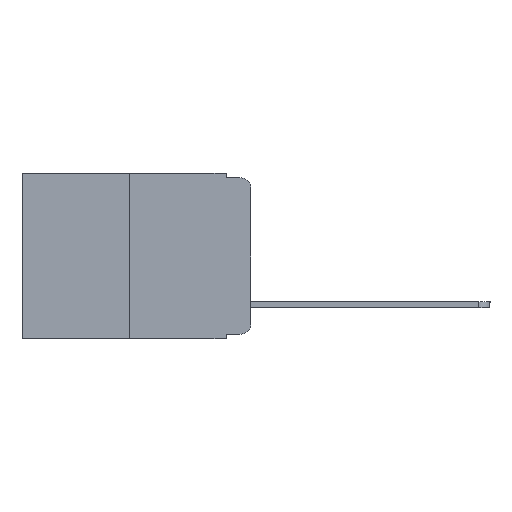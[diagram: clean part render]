
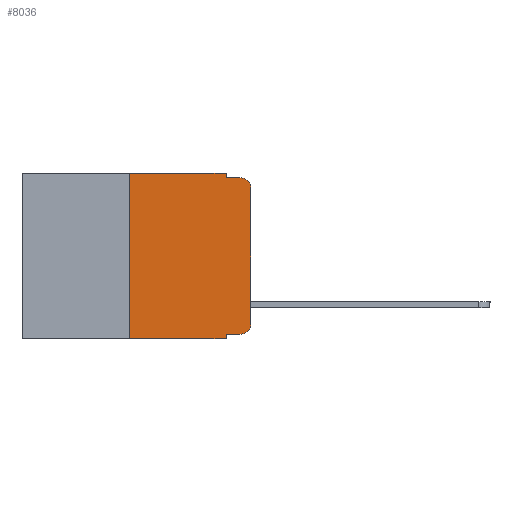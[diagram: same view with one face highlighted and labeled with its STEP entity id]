
A CAD part, left-side view. The second image highlights one B-rep face of the part: STEP entity #8036.
In plain terms, the highlighted planar face has unit normal (-1, 0, 0).
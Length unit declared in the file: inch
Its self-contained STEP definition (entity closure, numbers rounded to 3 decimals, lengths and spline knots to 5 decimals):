
#170 = CARTESIAN_POINT ( 'NONE',  ( 0., 0.473, 0. ) ) ;
#221 = PLANE ( 'NONE',  #8677 ) ;
#333 = LINE ( 'NONE', #6290, #721 ) ;
#510 = VECTOR ( 'NONE', #1348, 39.37008 ) ;
#678 = DIRECTION ( 'NONE',  ( 0., 0., -1. ) ) ;
#721 = VECTOR ( 'NONE', #17011, 39.37008 ) ;
#1108 = ORIENTED_EDGE ( 'NONE', *, *, #11790, .T. ) ;
#1348 = DIRECTION ( 'NONE',  ( 0., -1., 0. ) ) ;
#1428 = CARTESIAN_POINT ( 'NONE',  ( 0., 0., -0.03 ) ) ;
#1675 = VECTOR ( 'NONE', #11994, 39.37008 ) ;
#1897 = CARTESIAN_POINT ( 'NONE',  ( 0., 0.051, -0.343 ) ) ;
#2015 = CARTESIAN_POINT ( 'NONE',  ( 0., 0.25, -0.343 ) ) ;
#2225 = CARTESIAN_POINT ( 'NONE',  ( 0., 0.051, -0.01 ) ) ;
#2296 = LINE ( 'NONE', #15583, #2977 ) ;
#2380 = VERTEX_POINT ( 'NONE', #13948 ) ;
#2411 = DIRECTION ( 'NONE',  ( 0., 0., -1. ) ) ;
#2779 = CARTESIAN_POINT ( 'NONE',  ( 0., 0.25, 0. ) ) ;
#2977 = VECTOR ( 'NONE', #17019, 39.37008 ) ;
#2994 = CIRCLE ( 'NONE', #4972, 0.02 ) ;
#3076 = CARTESIAN_POINT ( 'NONE',  ( 0., 0.02, -0.333 ) ) ;
#3241 = CARTESIAN_POINT ( 'NONE',  ( 0., 0.051, -0.01 ) ) ;
#3662 = VECTOR ( 'NONE', #3894, 39.37008 ) ;
#3843 = ORIENTED_EDGE ( 'NONE', *, *, #6436, .F. ) ;
#3894 = DIRECTION ( 'NONE',  ( 0., 0., 1. ) ) ;
#4288 = DIRECTION ( 'NONE',  ( 0., 0., 1. ) ) ;
#4972 = AXIS2_PLACEMENT_3D ( 'NONE', #15851, #10313, #7544 ) ;
#5217 = VERTEX_POINT ( 'NONE', #17014 ) ;
#5223 = LINE ( 'NONE', #6297, #1675 ) ;
#5485 = CARTESIAN_POINT ( 'NONE',  ( 0., 0.051, 0. ) ) ;
#5678 = DIRECTION ( 'NONE',  ( 0., 0., -1. ) ) ;
#5856 = FACE_OUTER_BOUND ( 'NONE', #10238, .T. ) ;
#5994 = EDGE_CURVE ( 'NONE', #15196, #6560, #6374, .T. ) ;
#6131 = VECTOR ( 'NONE', #678, 39.37008 ) ;
#6213 = CARTESIAN_POINT ( 'NONE',  ( 0., 0., 0. ) ) ;
#6290 = CARTESIAN_POINT ( 'NONE',  ( 0., 0.473, -0.343 ) ) ;
#6297 = CARTESIAN_POINT ( 'NONE',  ( 0., 0.051, -0.333 ) ) ;
#6374 = CIRCLE ( 'NONE', #8653, 0.02 ) ;
#6408 = EDGE_CURVE ( 'NONE', #16904, #9557, #2994, .T. ) ;
#6436 = EDGE_CURVE ( 'NONE', #8267, #10161, #2296, .T. ) ;
#6558 = CARTESIAN_POINT ( 'NONE',  ( 0., 0., -0.313 ) ) ;
#6560 = VERTEX_POINT ( 'NONE', #6558 ) ;
#6779 = EDGE_CURVE ( 'NONE', #2380, #16649, #9028, .T. ) ;
#7008 = CARTESIAN_POINT ( 'NONE',  ( 0., 0.473, 0. ) ) ;
#7544 = DIRECTION ( 'NONE',  ( 0., 0., -1. ) ) ;
#8036 = ADVANCED_FACE ( 'NONE', ( #5856 ), #221, .F. ) ;
#8235 = ORIENTED_EDGE ( 'NONE', *, *, #12680, .F. ) ;
#8267 = VERTEX_POINT ( 'NONE', #5485 ) ;
#8609 = EDGE_CURVE ( 'NONE', #13499, #16649, #333, .T. ) ;
#8653 = AXIS2_PLACEMENT_3D ( 'NONE', #15605, #13169, #2411 ) ;
#8677 = AXIS2_PLACEMENT_3D ( 'NONE', #7008, #12427, #5678 ) ;
#8776 = ORIENTED_EDGE ( 'NONE', *, *, #11868, .T. ) ;
#8778 = ORIENTED_EDGE ( 'NONE', *, *, #11191, .F. ) ;
#9028 = LINE ( 'NONE', #11618, #6131 ) ;
#9557 = VERTEX_POINT ( 'NONE', #11331 ) ;
#9829 = DIRECTION ( 'NONE',  ( 0., -1., 0. ) ) ;
#10161 = VERTEX_POINT ( 'NONE', #2225 ) ;
#10238 = EDGE_LOOP ( 'NONE', ( #8776, #16117, #8235, #3843, #8778, #14400, #13300, #16002, #1108, #13656 ) ) ;
#10313 = DIRECTION ( 'NONE',  ( -1., 0., 0. ) ) ;
#10498 = VECTOR ( 'NONE', #9829, 39.37008 ) ;
#11062 = LINE ( 'NONE', #3241, #10498 ) ;
#11191 = EDGE_CURVE ( 'NONE', #5217, #8267, #16030, .T. ) ;
#11331 = CARTESIAN_POINT ( 'NONE',  ( 0., 0.02, -0.01 ) ) ;
#11618 = CARTESIAN_POINT ( 'NONE',  ( 0., 0.051, 0. ) ) ;
#11649 = VECTOR ( 'NONE', #4288, 39.37008 ) ;
#11790 = EDGE_CURVE ( 'NONE', #2380, #15196, #5223, .T. ) ;
#11868 = EDGE_CURVE ( 'NONE', #6560, #16904, #17186, .T. ) ;
#11994 = DIRECTION ( 'NONE',  ( 0., -1., 0. ) ) ;
#12415 = EDGE_CURVE ( 'NONE', #13499, #5217, #15073, .T. ) ;
#12427 = DIRECTION ( 'NONE',  ( 1., 0., 0. ) ) ;
#12680 = EDGE_CURVE ( 'NONE', #10161, #9557, #11062, .T. ) ;
#13169 = DIRECTION ( 'NONE',  ( -1., 0., 0. ) ) ;
#13300 = ORIENTED_EDGE ( 'NONE', *, *, #8609, .T. ) ;
#13499 = VERTEX_POINT ( 'NONE', #2015 ) ;
#13656 = ORIENTED_EDGE ( 'NONE', *, *, #5994, .T. ) ;
#13948 = CARTESIAN_POINT ( 'NONE',  ( 0., 0.051, -0.333 ) ) ;
#14400 = ORIENTED_EDGE ( 'NONE', *, *, #12415, .F. ) ;
#15073 = LINE ( 'NONE', #2779, #11649 ) ;
#15196 = VERTEX_POINT ( 'NONE', #3076 ) ;
#15583 = CARTESIAN_POINT ( 'NONE',  ( 0., 0.051, 0. ) ) ;
#15605 = CARTESIAN_POINT ( 'NONE',  ( 0., 0.02, -0.313 ) ) ;
#15851 = CARTESIAN_POINT ( 'NONE',  ( 0., 0.02, -0.03 ) ) ;
#16002 = ORIENTED_EDGE ( 'NONE', *, *, #6779, .F. ) ;
#16030 = LINE ( 'NONE', #170, #510 ) ;
#16117 = ORIENTED_EDGE ( 'NONE', *, *, #6408, .T. ) ;
#16649 = VERTEX_POINT ( 'NONE', #1897 ) ;
#16904 = VERTEX_POINT ( 'NONE', #1428 ) ;
#17011 = DIRECTION ( 'NONE',  ( 0., -1., 0. ) ) ;
#17014 = CARTESIAN_POINT ( 'NONE',  ( 0., 0.25, 0. ) ) ;
#17019 = DIRECTION ( 'NONE',  ( 0., 0., -1. ) ) ;
#17186 = LINE ( 'NONE', #6213, #3662 ) ;
